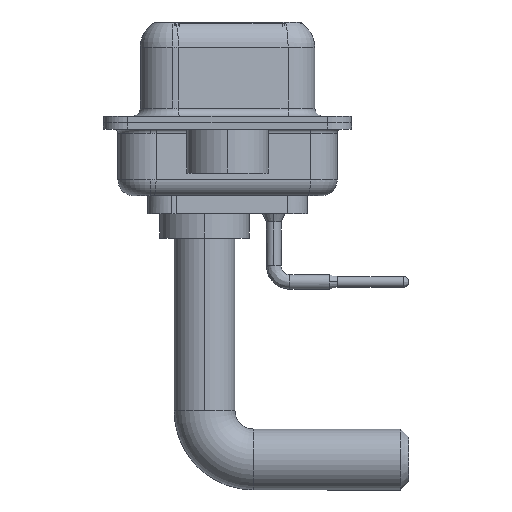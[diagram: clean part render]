
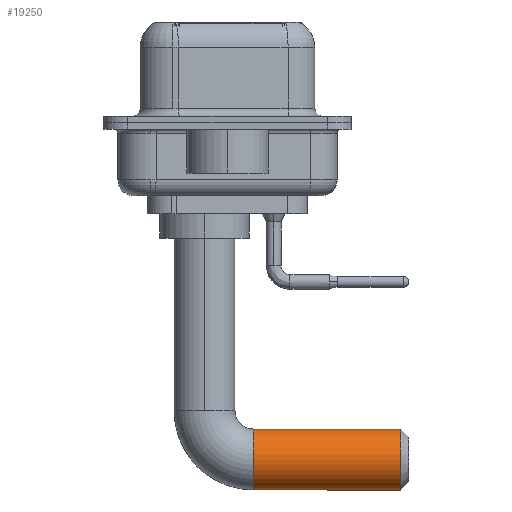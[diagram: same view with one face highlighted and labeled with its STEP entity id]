
A CAD part, left-side view. The second image highlights one B-rep face of the part: STEP entity #19250.
In plain terms, the highlighted cylindrical face has radius 1.875 mm (diameter 3.75 mm), a partial arc.
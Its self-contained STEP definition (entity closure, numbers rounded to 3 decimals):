
#181 = DIRECTION ( 'NONE',  ( 0., 0., -1. ) ) ;
#1575 = CIRCLE ( 'NONE', #6732, 1.875 ) ;
#1606 = EDGE_CURVE ( 'NONE', #12777, #4981, #13960, .T. ) ;
#1889 = FACE_OUTER_BOUND ( 'NONE', #7582, .T. ) ;
#2790 = EDGE_CURVE ( 'NONE', #3540, #4981, #8362, .T. ) ;
#3146 = DIRECTION ( 'NONE',  ( 0., -1., 0. ) ) ;
#3313 = CARTESIAN_POINT ( 'NONE',  ( 0., -3., -11.755 ) ) ;
#3540 = VERTEX_POINT ( 'NONE', #17857 ) ;
#3576 = LINE ( 'NONE', #16598, #14833 ) ;
#3621 = DIRECTION ( 'NONE',  ( 0., -1., 0. ) ) ;
#4043 = ORIENTED_EDGE ( 'NONE', *, *, #2790, .F. ) ;
#4079 = CARTESIAN_POINT ( 'NONE',  ( 0., -3., -13.63 ) ) ;
#4543 = ORIENTED_EDGE ( 'NONE', *, *, #11634, .T. ) ;
#4981 = VERTEX_POINT ( 'NONE', #8115 ) ;
#4994 = AXIS2_PLACEMENT_3D ( 'NONE', #18033, #3621, #181 ) ;
#6471 = VECTOR ( 'NONE', #18045, 1000. ) ;
#6732 = AXIS2_PLACEMENT_3D ( 'NONE', #4079, #17187, #8996 ) ;
#6857 = DIRECTION ( 'NONE',  ( 0., 0., -1. ) ) ;
#7582 = EDGE_LOOP ( 'NONE', ( #4043, #7896, #4543, #12497 ) ) ;
#7896 = ORIENTED_EDGE ( 'NONE', *, *, #17283, .T. ) ;
#8082 = VERTEX_POINT ( 'NONE', #9256 ) ;
#8115 = CARTESIAN_POINT ( 'NONE',  ( 0., -12.07, -11.755 ) ) ;
#8362 = LINE ( 'NONE', #3313, #6471 ) ;
#8996 = DIRECTION ( 'NONE',  ( -1., 0., 0. ) ) ;
#9256 = CARTESIAN_POINT ( 'NONE',  ( 0., -3., -15.505 ) ) ;
#11556 = AXIS2_PLACEMENT_3D ( 'NONE', #13409, #15042, #6857 ) ;
#11584 = CYLINDRICAL_SURFACE ( 'NONE', #4994, 1.875 ) ;
#11634 = EDGE_CURVE ( 'NONE', #8082, #12777, #3576, .T. ) ;
#12497 = ORIENTED_EDGE ( 'NONE', *, *, #1606, .T. ) ;
#12777 = VERTEX_POINT ( 'NONE', #13704 ) ;
#13409 = CARTESIAN_POINT ( 'NONE',  ( 0., -12.07, -13.63 ) ) ;
#13704 = CARTESIAN_POINT ( 'NONE',  ( 0., -12.07, -15.505 ) ) ;
#13960 = CIRCLE ( 'NONE', #11556, 1.875 ) ;
#14833 = VECTOR ( 'NONE', #3146, 1000. ) ;
#15042 = DIRECTION ( 'NONE',  ( 0., 1., 0. ) ) ;
#16598 = CARTESIAN_POINT ( 'NONE',  ( 0., -3., -15.505 ) ) ;
#17187 = DIRECTION ( 'NONE',  ( 0., -1., 0. ) ) ;
#17283 = EDGE_CURVE ( 'NONE', #3540, #8082, #1575, .T. ) ;
#17857 = CARTESIAN_POINT ( 'NONE',  ( 0., -3., -11.755 ) ) ;
#18033 = CARTESIAN_POINT ( 'NONE',  ( 0., -3., -13.63 ) ) ;
#18045 = DIRECTION ( 'NONE',  ( 0., -1., 0. ) ) ;
#19250 = ADVANCED_FACE ( 'NONE', ( #1889 ), #11584, .T. ) ;
